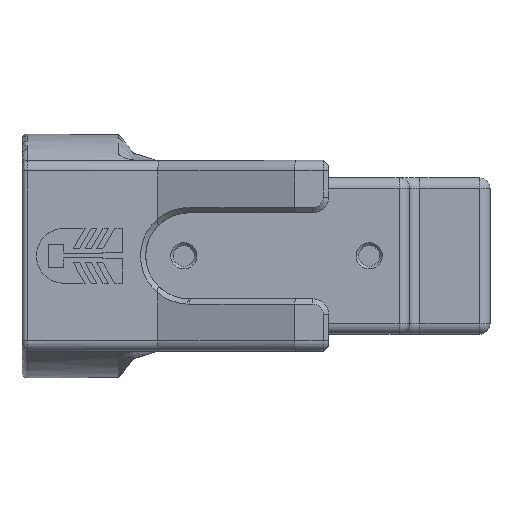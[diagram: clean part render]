
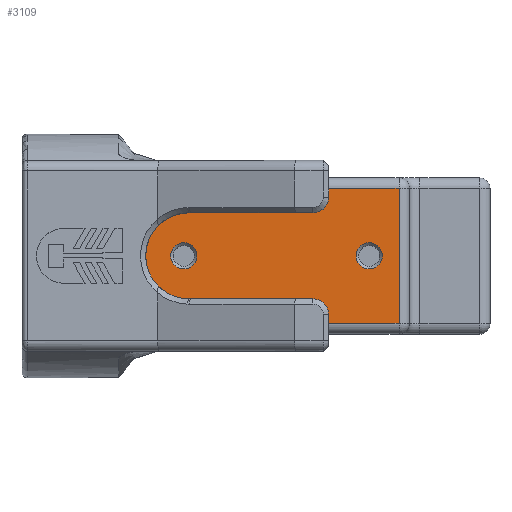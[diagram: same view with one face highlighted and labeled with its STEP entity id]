
A CAD part, top view. The second image highlights one B-rep face of the part: STEP entity #3109.
In plain terms, the highlighted planar face has unit normal (0, 0, 1).
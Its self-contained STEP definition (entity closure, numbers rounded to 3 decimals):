
#57=FACE_BOUND('',#435,.T.);
#58=FACE_BOUND('',#436,.T.);
#64=PLANE('',#3313);
#152=CIRCLE('',#3311,2.5);
#154=CIRCLE('',#3314,3.);
#155=CIRCLE('',#3315,8.24);
#156=CIRCLE('',#3316,3.);
#157=CIRCLE('',#3317,2.5);
#250=FACE_OUTER_BOUND('',#434,.T.);
#434=EDGE_LOOP('',(#2145,#2146,#2147,#2148,#2149,#2150,#2151,#2152,#2153,
#2154));
#435=EDGE_LOOP('',(#2155));
#436=EDGE_LOOP('',(#2156));
#726=LINE('',#5532,#1009);
#727=LINE('',#5534,#1010);
#728=LINE('',#5536,#1011);
#729=LINE('',#5538,#1012);
#730=LINE('',#5542,#1013);
#731=LINE('',#5546,#1014);
#732=LINE('',#5549,#1015);
#1009=VECTOR('',#3631,10.);
#1010=VECTOR('',#3632,10.);
#1011=VECTOR('',#3633,10.);
#1012=VECTOR('',#3634,10.3);
#1013=VECTOR('',#3637,10.3);
#1014=VECTOR('',#3640,1030.);
#1015=VECTOR('',#3643,10.3);
#1332=VERTEX_POINT('',#5524);
#1334=VERTEX_POINT('',#5530);
#1335=VERTEX_POINT('',#5531);
#1336=VERTEX_POINT('',#5533);
#1337=VERTEX_POINT('',#5535);
#1338=VERTEX_POINT('',#5537);
#1339=VERTEX_POINT('',#5539);
#1340=VERTEX_POINT('',#5541);
#1341=VERTEX_POINT('',#5543);
#1342=VERTEX_POINT('',#5545);
#1343=VERTEX_POINT('',#5547);
#1344=VERTEX_POINT('',#5550);
#1648=EDGE_CURVE('',#1332,#1332,#152,.T.);
#1651=EDGE_CURVE('',#1334,#1335,#726,.T.);
#1652=EDGE_CURVE('',#1336,#1334,#727,.T.);
#1653=EDGE_CURVE('',#1337,#1336,#728,.T.);
#1654=EDGE_CURVE('',#1337,#1338,#729,.T.);
#1655=EDGE_CURVE('',#1339,#1338,#154,.F.);
#1656=EDGE_CURVE('',#1339,#1340,#730,.T.);
#1657=EDGE_CURVE('',#1340,#1341,#155,.T.);
#1658=EDGE_CURVE('',#1341,#1342,#731,.T.);
#1659=EDGE_CURVE('',#1343,#1342,#156,.F.);
#1660=EDGE_CURVE('',#1343,#1335,#732,.T.);
#1661=EDGE_CURVE('',#1344,#1344,#157,.T.);
#2145=ORIENTED_EDGE('',*,*,#1651,.F.);
#2146=ORIENTED_EDGE('',*,*,#1652,.F.);
#2147=ORIENTED_EDGE('',*,*,#1653,.F.);
#2148=ORIENTED_EDGE('',*,*,#1654,.T.);
#2149=ORIENTED_EDGE('',*,*,#1655,.F.);
#2150=ORIENTED_EDGE('',*,*,#1656,.T.);
#2151=ORIENTED_EDGE('',*,*,#1657,.T.);
#2152=ORIENTED_EDGE('',*,*,#1658,.T.);
#2153=ORIENTED_EDGE('',*,*,#1659,.F.);
#2154=ORIENTED_EDGE('',*,*,#1660,.T.);
#2155=ORIENTED_EDGE('',*,*,#1661,.F.);
#2156=ORIENTED_EDGE('',*,*,#1648,.F.);
#3109=ADVANCED_FACE('',(#250,#57,#58),#64,.T.);
#3311=AXIS2_PLACEMENT_3D('',#5525,#3624,#3625);
#3313=AXIS2_PLACEMENT_3D('',#5529,#3629,#3630);
#3314=AXIS2_PLACEMENT_3D('',#5540,#3635,#3636);
#3315=AXIS2_PLACEMENT_3D('',#5544,#3638,#3639);
#3316=AXIS2_PLACEMENT_3D('',#5548,#3641,#3642);
#3317=AXIS2_PLACEMENT_3D('',#5551,#3644,#3645);
#3624=DIRECTION('center_axis',(0.,0.,
1.));
#3625=DIRECTION('ref_axis',(-1.,0.,0.));
#3629=DIRECTION('center_axis',(0.,0.,
1.));
#3630=DIRECTION('ref_axis',(-1.,0.,0.));
#3631=DIRECTION('',(-1.,0.,0.));
#3632=DIRECTION('',(0.,-1.,0.));
#3633=DIRECTION('',(1.,0.,0.));
#3634=DIRECTION('',(0.,-1.,0.));
#3635=DIRECTION('center_axis',(0.,0.,
-1.));
#3636=DIRECTION('ref_axis',(0.707,-0.707,0.));
#3637=DIRECTION('',(-1.,0.,0.));
#3638=DIRECTION('center_axis',(0.,0.,
1.));
#3639=DIRECTION('ref_axis',(-0.707,0.707,0.));
#3640=DIRECTION('',(1.,0.,0.));
#3641=DIRECTION('center_axis',(0.,0.,
-1.));
#3642=DIRECTION('ref_axis',(0.707,0.707,0.));
#3643=DIRECTION('',(0.,-1.,0.));
#3644=DIRECTION('center_axis',(0.,0.,
1.));
#3645=DIRECTION('ref_axis',(-1.,0.,0.));
#5524=CARTESIAN_POINT('',(260.899,115.788,16.674));
#5525=CARTESIAN_POINT('Origin',(258.399,115.788,16.674));
#5529=CARTESIAN_POINT('Origin',(250.629,131.238,16.674));
#5530=CARTESIAN_POINT('',(264.109,102.838,16.674));
#5531=CARTESIAN_POINT('',(250.629,102.838,16.674));
#5532=CARTESIAN_POINT('',(258.869,102.838,16.674));
#5533=CARTESIAN_POINT('',(264.109,128.738,16.674));
#5534=CARTESIAN_POINT('',(264.109,131.238,16.674));
#5535=CARTESIAN_POINT('',(250.629,128.738,16.674));
#5536=CARTESIAN_POINT('',(258.869,128.738,16.674));
#5537=CARTESIAN_POINT('',(250.629,127.028,16.674));
#5538=CARTESIAN_POINT('',(250.629,128.663,16.674));
#5539=CARTESIAN_POINT('',(247.629,124.028,16.674));
#5540=CARTESIAN_POINT('Origin',(247.629,127.028,16.674));
#5541=CARTESIAN_POINT('',(223.849,124.028,16.674));
#5542=CARTESIAN_POINT('',(223.849,124.028,16.674));
#5543=CARTESIAN_POINT('',(223.849,107.548,16.674));
#5544=CARTESIAN_POINT('Origin',(223.849,115.788,16.674));
#5545=CARTESIAN_POINT('',(247.629,107.548,16.674));
#5546=CARTESIAN_POINT('',(223.849,107.548,16.674));
#5547=CARTESIAN_POINT('',(250.629,104.548,16.674));
#5548=CARTESIAN_POINT('Origin',(247.629,104.548,16.674));
#5549=CARTESIAN_POINT('',(250.629,118.363,16.674));
#5550=CARTESIAN_POINT('',(225.399,115.788,16.674));
#5551=CARTESIAN_POINT('Origin',(222.899,115.788,16.674));
